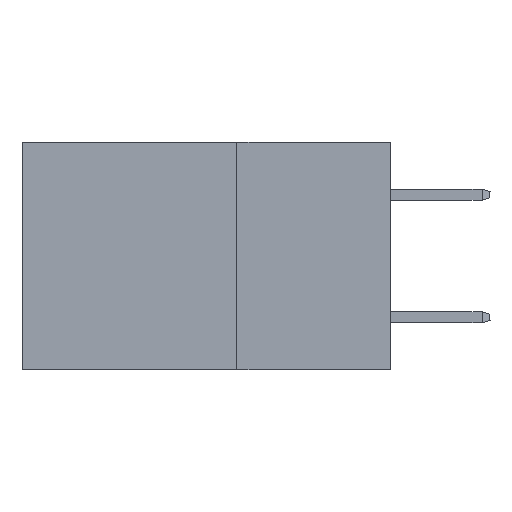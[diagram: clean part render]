
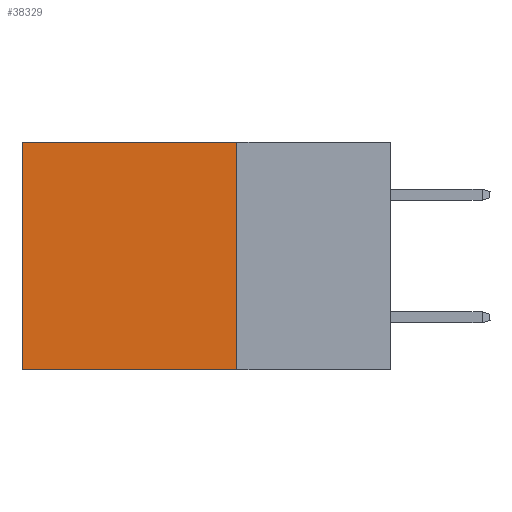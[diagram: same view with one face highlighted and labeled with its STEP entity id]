
A CAD part, left-side view. The second image highlights one B-rep face of the part: STEP entity #38329.
In plain terms, the highlighted planar face has unit normal (-1, 0, 0).
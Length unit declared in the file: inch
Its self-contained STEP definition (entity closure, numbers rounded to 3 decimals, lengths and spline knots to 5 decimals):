
#1935 = EDGE_CURVE ( 'NONE', #35642, #46341, #23548, .T. ) ;
#2292 = LINE ( 'NONE', #40557, #37250 ) ;
#3745 = VECTOR ( 'NONE', #15306, 39.37008 ) ;
#3900 = EDGE_CURVE ( 'NONE', #35642, #43843, #2292, .T. ) ;
#4760 = DIRECTION ( 'NONE',  ( 0., 0., -1. ) ) ;
#4889 = EDGE_LOOP ( 'NONE', ( #18041, #26916, #15780, #44835 ) ) ;
#8242 = CARTESIAN_POINT ( 'NONE',  ( 0.2875, 0.6, -0.37 ) ) ;
#8519 = CARTESIAN_POINT ( 'NONE',  ( 0.2875, 0.25, 0. ) ) ;
#12141 = DIRECTION ( 'NONE',  ( 0., 0., -1. ) ) ;
#12280 = CARTESIAN_POINT ( 'NONE',  ( 0.2875, 0.25, -0.37 ) ) ;
#12375 = CARTESIAN_POINT ( 'NONE',  ( 0.2875, 0.25, 0. ) ) ;
#13385 = LINE ( 'NONE', #33380, #3745 ) ;
#15306 = DIRECTION ( 'NONE',  ( 0., 0., -1. ) ) ;
#15532 = EDGE_CURVE ( 'NONE', #43843, #17975, #42985, .T. ) ;
#15780 = ORIENTED_EDGE ( 'NONE', *, *, #3900, .F. ) ;
#16711 = CARTESIAN_POINT ( 'NONE',  ( 0.2875, 0.25, -0.37 ) ) ;
#17975 = VERTEX_POINT ( 'NONE', #8242 ) ;
#18041 = ORIENTED_EDGE ( 'NONE', *, *, #18696, .T. ) ;
#18696 = EDGE_CURVE ( 'NONE', #46341, #17975, #13385, .T. ) ;
#23117 = DIRECTION ( 'NONE',  ( 0., 1., 0. ) ) ;
#23548 = LINE ( 'NONE', #12375, #30775 ) ;
#26916 = ORIENTED_EDGE ( 'NONE', *, *, #15532, .F. ) ;
#26919 = DIRECTION ( 'NONE',  ( 0., 1., 0. ) ) ;
#28036 = CARTESIAN_POINT ( 'NONE',  ( 0.2875, 0.6, 0. ) ) ;
#30775 = VECTOR ( 'NONE', #26919, 39.37008 ) ;
#33380 = CARTESIAN_POINT ( 'NONE',  ( 0.2875, 0.6, 0. ) ) ;
#33552 = VECTOR ( 'NONE', #23117, 39.37008 ) ;
#33718 = DIRECTION ( 'NONE',  ( 1., 0., 0. ) ) ;
#35642 = VERTEX_POINT ( 'NONE', #46036 ) ;
#37250 = VECTOR ( 'NONE', #4760, 39.37008 ) ;
#38329 = ADVANCED_FACE ( 'NONE', ( #46370 ), #44271, .F. ) ;
#40557 = CARTESIAN_POINT ( 'NONE',  ( 0.2875, 0.25, 0. ) ) ;
#42985 = LINE ( 'NONE', #12280, #33552 ) ;
#43843 = VERTEX_POINT ( 'NONE', #16711 ) ;
#44137 = AXIS2_PLACEMENT_3D ( 'NONE', #8519, #33718, #12141 ) ;
#44271 = PLANE ( 'NONE',  #44137 ) ;
#44835 = ORIENTED_EDGE ( 'NONE', *, *, #1935, .T. ) ;
#46036 = CARTESIAN_POINT ( 'NONE',  ( 0.2875, 0.25, 0. ) ) ;
#46341 = VERTEX_POINT ( 'NONE', #28036 ) ;
#46370 = FACE_OUTER_BOUND ( 'NONE', #4889, .T. ) ;
